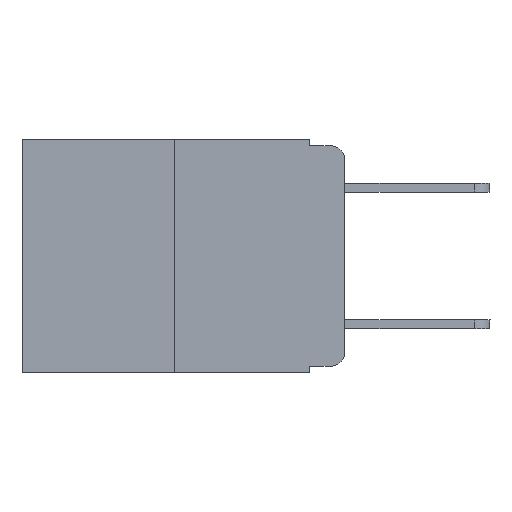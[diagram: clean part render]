
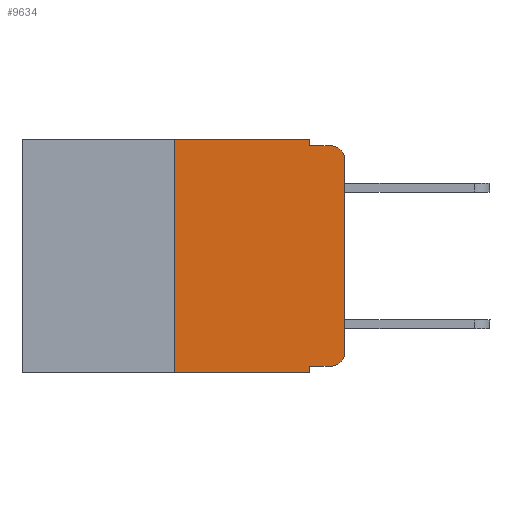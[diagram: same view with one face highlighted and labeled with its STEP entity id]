
A CAD part, left-side view. The second image highlights one B-rep face of the part: STEP entity #9634.
In plain terms, the highlighted planar face has unit normal (-1, 0, 0).
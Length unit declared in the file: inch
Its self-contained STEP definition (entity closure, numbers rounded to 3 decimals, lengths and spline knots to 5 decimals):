
#79 = EDGE_CURVE ( 'NONE', #14640, #13151, #7366, .T. ) ;
#131 = CARTESIAN_POINT ( 'NONE',  ( 0., 0.473, -0.343 ) ) ;
#301 = LINE ( 'NONE', #7259, #3541 ) ;
#383 = VECTOR ( 'NONE', #13623, 39.37008 ) ;
#426 = VECTOR ( 'NONE', #10891, 39.37008 ) ;
#458 = PLANE ( 'NONE',  #15473 ) ;
#480 = CARTESIAN_POINT ( 'NONE',  ( 0., 0.02, -0.313 ) ) ;
#511 = EDGE_CURVE ( 'NONE', #15180, #9740, #9612, .T. ) ;
#518 = CARTESIAN_POINT ( 'NONE',  ( 0., 0.02, -0.01 ) ) ;
#816 = CARTESIAN_POINT ( 'NONE',  ( 0., 0.25, -0.343 ) ) ;
#985 = CARTESIAN_POINT ( 'NONE',  ( 0., 0.25, 0. ) ) ;
#1024 = CARTESIAN_POINT ( 'NONE',  ( 0., 0.02, -0.03 ) ) ;
#1368 = DIRECTION ( 'NONE',  ( 0., 0., 1. ) ) ;
#1521 = ORIENTED_EDGE ( 'NONE', *, *, #511, .F. ) ;
#1928 = EDGE_CURVE ( 'NONE', #4542, #10880, #301, .T. ) ;
#2301 = ORIENTED_EDGE ( 'NONE', *, *, #14618, .T. ) ;
#2480 = CARTESIAN_POINT ( 'NONE',  ( 0., 0.051, 0. ) ) ;
#3001 = CARTESIAN_POINT ( 'NONE',  ( 0., 0.25, 0. ) ) ;
#3382 = VECTOR ( 'NONE', #3540, 39.37008 ) ;
#3540 = DIRECTION ( 'NONE',  ( 0., 0., -1. ) ) ;
#3541 = VECTOR ( 'NONE', #8349, 39.37008 ) ;
#3857 = VECTOR ( 'NONE', #1368, 39.37008 ) ;
#3896 = CIRCLE ( 'NONE', #9939, 0.02 ) ;
#3898 = EDGE_CURVE ( 'NONE', #4257, #4542, #8511, .T. ) ;
#3935 = VERTEX_POINT ( 'NONE', #985 ) ;
#3989 = CARTESIAN_POINT ( 'NONE',  ( 0., 0.473, 0. ) ) ;
#4096 = CARTESIAN_POINT ( 'NONE',  ( 0., 0.473, 0. ) ) ;
#4121 = CIRCLE ( 'NONE', #14675, 0.02 ) ;
#4256 = DIRECTION ( 'NONE',  ( 0., 0., 1. ) ) ;
#4257 = VERTEX_POINT ( 'NONE', #10191 ) ;
#4261 = CARTESIAN_POINT ( 'NONE',  ( 0., 0., -0.03 ) ) ;
#4325 = LINE ( 'NONE', #3001, #10133 ) ;
#4542 = VERTEX_POINT ( 'NONE', #9796 ) ;
#4746 = EDGE_CURVE ( 'NONE', #11090, #3935, #4325, .T. ) ;
#5213 = EDGE_LOOP ( 'NONE', ( #5510, #10823, #13043, #8626, #6527, #5878, #8576, #1521, #2301, #11498 ) ) ;
#5244 = DIRECTION ( 'NONE',  ( 0., -1., 0. ) ) ;
#5270 = DIRECTION ( 'NONE',  ( -1., 0., 0. ) ) ;
#5510 = ORIENTED_EDGE ( 'NONE', *, *, #79, .T. ) ;
#5674 = CARTESIAN_POINT ( 'NONE',  ( 0., 0.051, -0.333 ) ) ;
#5878 = ORIENTED_EDGE ( 'NONE', *, *, #4746, .F. ) ;
#5905 = CARTESIAN_POINT ( 'NONE',  ( 0., 0.02, -0.333 ) ) ;
#5939 = VECTOR ( 'NONE', #5244, 39.37008 ) ;
#6297 = VERTEX_POINT ( 'NONE', #5905 ) ;
#6527 = ORIENTED_EDGE ( 'NONE', *, *, #11941, .F. ) ;
#7224 = VECTOR ( 'NONE', #9305, 39.37008 ) ;
#7259 = CARTESIAN_POINT ( 'NONE',  ( 0., 0.051, -0.01 ) ) ;
#7366 = LINE ( 'NONE', #12156, #3857 ) ;
#7442 = EDGE_CURVE ( 'NONE', #13151, #10880, #4121, .T. ) ;
#8347 = CARTESIAN_POINT ( 'NONE',  ( 0., 0.051, -0.333 ) ) ;
#8349 = DIRECTION ( 'NONE',  ( 0., -1., 0. ) ) ;
#8511 = LINE ( 'NONE', #2480, #426 ) ;
#8576 = ORIENTED_EDGE ( 'NONE', *, *, #9626, .T. ) ;
#8626 = ORIENTED_EDGE ( 'NONE', *, *, #3898, .F. ) ;
#8736 = LINE ( 'NONE', #131, #5939 ) ;
#8912 = LINE ( 'NONE', #4096, #383 ) ;
#9305 = DIRECTION ( 'NONE',  ( 0., -1., 0. ) ) ;
#9612 = LINE ( 'NONE', #10736, #3382 ) ;
#9626 = EDGE_CURVE ( 'NONE', #11090, #9740, #8736, .T. ) ;
#9634 = ADVANCED_FACE ( 'NONE', ( #11022 ), #458, .F. ) ;
#9740 = VERTEX_POINT ( 'NONE', #11464 ) ;
#9796 = CARTESIAN_POINT ( 'NONE',  ( 0., 0.051, -0.01 ) ) ;
#9939 = AXIS2_PLACEMENT_3D ( 'NONE', #480, #5270, #10077 ) ;
#10077 = DIRECTION ( 'NONE',  ( 0., 0., -1. ) ) ;
#10133 = VECTOR ( 'NONE', #4256, 39.37008 ) ;
#10191 = CARTESIAN_POINT ( 'NONE',  ( 0., 0.051, 0. ) ) ;
#10736 = CARTESIAN_POINT ( 'NONE',  ( 0., 0.051, 0. ) ) ;
#10823 = ORIENTED_EDGE ( 'NONE', *, *, #7442, .T. ) ;
#10880 = VERTEX_POINT ( 'NONE', #518 ) ;
#10891 = DIRECTION ( 'NONE',  ( 0., 0., -1. ) ) ;
#10963 = CARTESIAN_POINT ( 'NONE',  ( 0., 0., -0.313 ) ) ;
#11022 = FACE_OUTER_BOUND ( 'NONE', #5213, .T. ) ;
#11090 = VERTEX_POINT ( 'NONE', #816 ) ;
#11464 = CARTESIAN_POINT ( 'NONE',  ( 0., 0.051, -0.343 ) ) ;
#11498 = ORIENTED_EDGE ( 'NONE', *, *, #13574, .T. ) ;
#11755 = DIRECTION ( 'NONE',  ( -1., 0., 0. ) ) ;
#11941 = EDGE_CURVE ( 'NONE', #3935, #4257, #8912, .T. ) ;
#12156 = CARTESIAN_POINT ( 'NONE',  ( 0., 0., 0. ) ) ;
#13043 = ORIENTED_EDGE ( 'NONE', *, *, #1928, .F. ) ;
#13151 = VERTEX_POINT ( 'NONE', #4261 ) ;
#13429 = DIRECTION ( 'NONE',  ( 0., 0., -1. ) ) ;
#13574 = EDGE_CURVE ( 'NONE', #6297, #14640, #3896, .T. ) ;
#13623 = DIRECTION ( 'NONE',  ( 0., -1., 0. ) ) ;
#13661 = DIRECTION ( 'NONE',  ( 1., 0., 0. ) ) ;
#14618 = EDGE_CURVE ( 'NONE', #15180, #6297, #15177, .T. ) ;
#14640 = VERTEX_POINT ( 'NONE', #10963 ) ;
#14675 = AXIS2_PLACEMENT_3D ( 'NONE', #1024, #11755, #15503 ) ;
#15177 = LINE ( 'NONE', #5674, #7224 ) ;
#15180 = VERTEX_POINT ( 'NONE', #8347 ) ;
#15473 = AXIS2_PLACEMENT_3D ( 'NONE', #3989, #13661, #13429 ) ;
#15503 = DIRECTION ( 'NONE',  ( 0., 0., -1. ) ) ;
